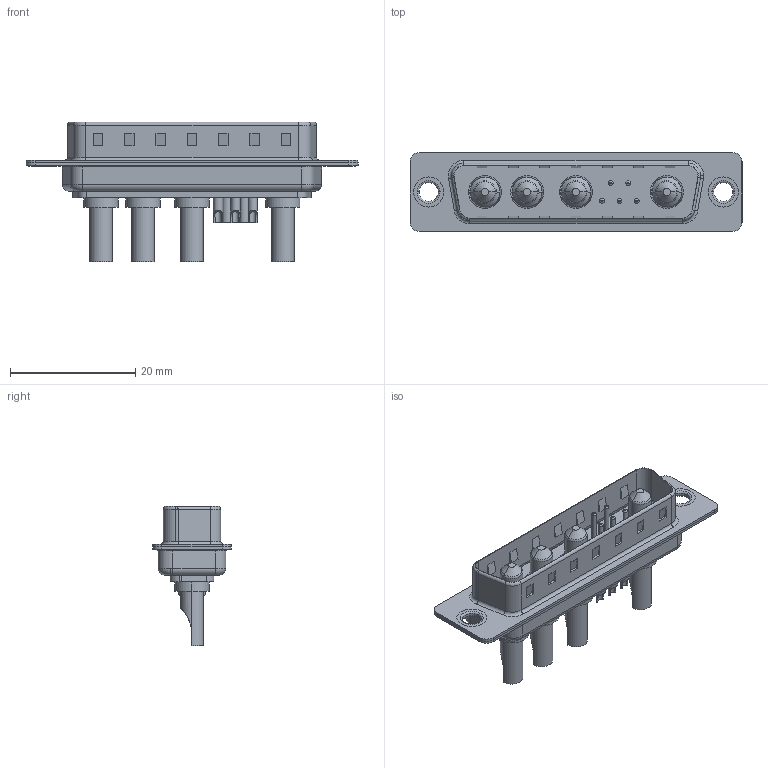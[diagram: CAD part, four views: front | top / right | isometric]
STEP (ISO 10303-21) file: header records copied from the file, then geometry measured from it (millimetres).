
FILE_DESCRIPTION (( 'STEP AP203' ), '1' );
FILE_NAME ('627-9W4-222-2T1.STEP', '2019-05-26T03:06:38', ( '' ), ( '' ), 'SwSTEP 2.0', 'SolidWorks 2016', '' );
FILE_SCHEMA (( 'CONFIG_CONTROL_DESIGN' ));
Length unit declared in the file: millimetre
Products named in the file (8): 627Combo Shell Rear_25 Contacts; 627Combo Shell Front_25 Contacts; 627Combo Thru Hole Rivet; Power Pin_20A SC; 627-9W4-222-2T1; 627Combo Contact Row 1_22; 627Combo Contact Row 2_22; 627Combo Housing_9W4
Assembly tree (14 placements, depth 2):
  627-9W4-222-2T1
    627Combo Housing_9W4
    627Combo Shell Rear_25 Contacts
    627Combo Shell Front_25 Contacts
    627Combo Thru Hole Rivet  x2
    Power Pin_20A SC  x4
    627Combo Contact Row 1_22  x2
    627Combo Contact Row 2_22  x3
Bounding box: 53 x 12.6 x 22.3 mm (x, y, z)
Volume: 2974.8 mm3; surface area: 6934 mm2
Topology: 18 solids, 18 shells, 719 faces, 1703 edges, 1045 vertices
Faces by surface type: cylinder 289, plane 268, torus 116, cone 38, bspline 8
Entity records: 15646 total; most frequent: CARTESIAN_POINT 2687, DIRECTION 2647, ORIENTED_EDGE 2374, EDGE_CURVE 1187, AXIS2_PLACEMENT_3D 999, VERTEX_POINT 745, LINE 649, VECTOR 649
